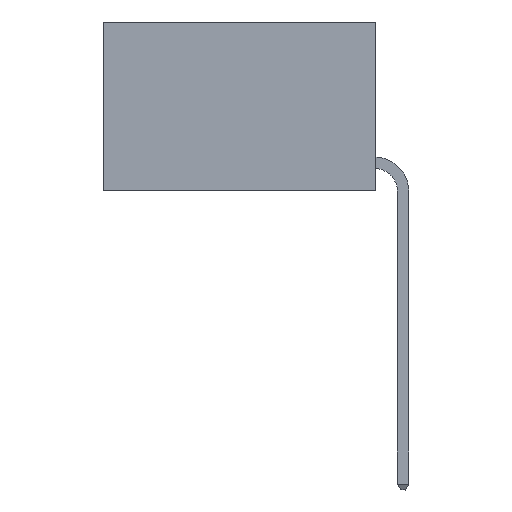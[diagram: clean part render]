
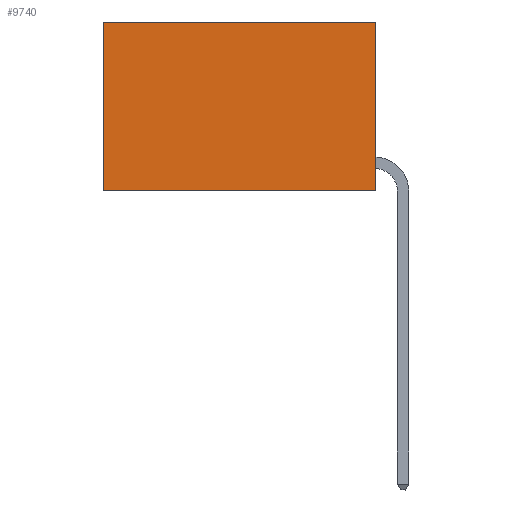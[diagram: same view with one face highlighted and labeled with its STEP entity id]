
A CAD part, left-side view. The second image highlights one B-rep face of the part: STEP entity #9740.
In plain terms, the highlighted planar face has unit normal (-1, 0, 0).
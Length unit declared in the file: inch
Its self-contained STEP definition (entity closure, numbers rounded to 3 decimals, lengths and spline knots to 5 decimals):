
#22 = EDGE_CURVE ( 'NONE', #13947, #6404, #1924, .T. ) ;
#114 = EDGE_CURVE ( 'NONE', #9491, #11034, #23508, .T. ) ;
#181 = CARTESIAN_POINT ( 'NONE',  ( 0.2625, 0.6, -0.37 ) ) ;
#453 = ORIENTED_EDGE ( 'NONE', *, *, #22, .F. ) ;
#813 = DIRECTION ( 'NONE',  ( 0., 1., 0. ) ) ;
#1307 = FACE_OUTER_BOUND ( 'NONE', #3326, .T. ) ;
#1703 = LINE ( 'NONE', #11321, #25437 ) ;
#1924 = LINE ( 'NONE', #2085, #13488 ) ;
#2085 = CARTESIAN_POINT ( 'NONE',  ( 0.2625, 0., -0.37 ) ) ;
#2161 = PLANE ( 'NONE',  #22645 ) ;
#3326 = EDGE_LOOP ( 'NONE', ( #6318, #453, #8148, #5449 ) ) ;
#4503 = DIRECTION ( 'NONE',  ( 1., 0., 0. ) ) ;
#5449 = ORIENTED_EDGE ( 'NONE', *, *, #114, .T. ) ;
#5923 = VECTOR ( 'NONE', #813, 39.37008 ) ;
#6318 = ORIENTED_EDGE ( 'NONE', *, *, #9107, .T. ) ;
#6404 = VERTEX_POINT ( 'NONE', #181 ) ;
#7074 = LINE ( 'NONE', #25908, #19294 ) ;
#8148 = ORIENTED_EDGE ( 'NONE', *, *, #11106, .F. ) ;
#9107 = EDGE_CURVE ( 'NONE', #11034, #6404, #1703, .T. ) ;
#9491 = VERTEX_POINT ( 'NONE', #12685 ) ;
#9602 = CARTESIAN_POINT ( 'NONE',  ( 0.2625, 0.6, 0. ) ) ;
#9740 = ADVANCED_FACE ( 'NONE', ( #1307 ), #2161, .F. ) ;
#11034 = VERTEX_POINT ( 'NONE', #9602 ) ;
#11106 = EDGE_CURVE ( 'NONE', #9491, #13947, #7074, .T. ) ;
#11321 = CARTESIAN_POINT ( 'NONE',  ( 0.2625, 0.6, 0. ) ) ;
#12206 = DIRECTION ( 'NONE',  ( 0., 0., -1. ) ) ;
#12685 = CARTESIAN_POINT ( 'NONE',  ( 0.2625, 0., 0. ) ) ;
#13488 = VECTOR ( 'NONE', #18710, 39.37008 ) ;
#13947 = VERTEX_POINT ( 'NONE', #29530 ) ;
#14596 = CARTESIAN_POINT ( 'NONE',  ( 0.2625, 0., 0. ) ) ;
#18249 = DIRECTION ( 'NONE',  ( 0., 0., -1. ) ) ;
#18314 = CARTESIAN_POINT ( 'NONE',  ( 0.2625, 0., 0. ) ) ;
#18710 = DIRECTION ( 'NONE',  ( 0., 1., 0. ) ) ;
#19294 = VECTOR ( 'NONE', #12206, 39.37008 ) ;
#20610 = DIRECTION ( 'NONE',  ( 0., 0., -1. ) ) ;
#22645 = AXIS2_PLACEMENT_3D ( 'NONE', #18314, #4503, #20610 ) ;
#23508 = LINE ( 'NONE', #14596, #5923 ) ;
#25437 = VECTOR ( 'NONE', #18249, 39.37008 ) ;
#25908 = CARTESIAN_POINT ( 'NONE',  ( 0.2625, 0., 0. ) ) ;
#29530 = CARTESIAN_POINT ( 'NONE',  ( 0.2625, 0., -0.37 ) ) ;
